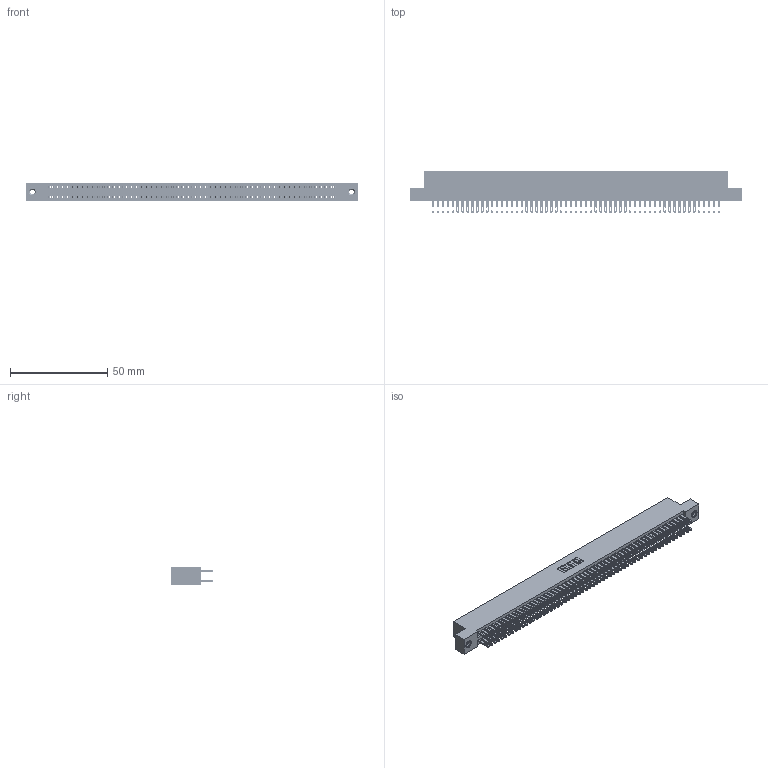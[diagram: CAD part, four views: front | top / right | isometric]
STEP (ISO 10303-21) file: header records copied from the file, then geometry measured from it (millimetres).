
FILE_DESCRIPTION (( 'STEP AP203' ), '1' );
FILE_NAME ('345-118-500-208.STEP', '2018-10-18T20:45:47', ( '' ), ( '' ), 'SwSTEP 2.0', 'SolidWorks 2016', '' );
FILE_SCHEMA (( 'CONFIG_CONTROL_DESIGN' ));
Length unit declared in the file: inch
Products named in the file (4): 345 Part_Flush Mounting Lugs - 0.156 Dia-TI; 345-292-001_345-293-100; 345-250-001_345-250-003-102; 345-118-500-208
Assembly tree (121 placements, depth 2):
  345-118-500-208
    345 Part_Flush Mounting Lugs - 0.156 Dia-TI
    345-292-001_345-293-100  x118
    345-250-001_345-250-003-102  x2
Bounding box: 171.07 x 21.51 x 9.4 mm (x, y, z)
Volume: 17129.7 mm3; surface area: 26866.8 mm2
Topology: 121 solids, 121 shells, 5614 faces, 17115 edges, 11402 vertices
Faces by surface type: plane 3298, cylinder 2300, cone 12, torus 4
Entity records: 45120 total; most frequent: CARTESIAN_POINT 7527, ORIENTED_EDGE 7454, DIRECTION 6645, EDGE_CURVE 3727, LINE 3335, VECTOR 3335, VERTEX_POINT 2480, AXIS2_PLACEMENT_3D 1655
